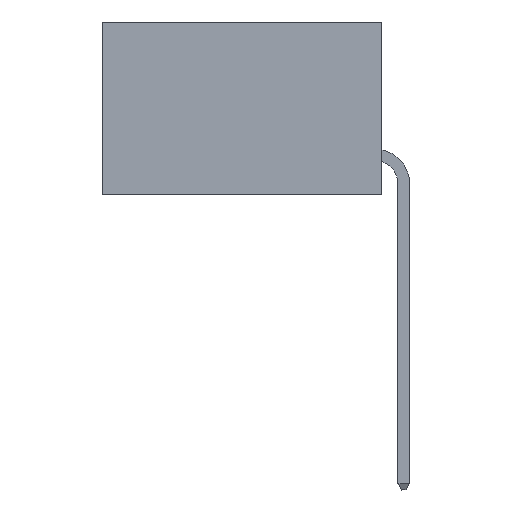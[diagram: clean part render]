
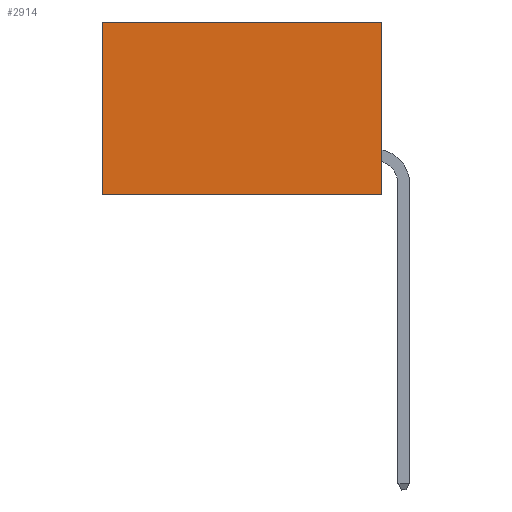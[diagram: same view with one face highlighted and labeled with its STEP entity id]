
A CAD part, left-side view. The second image highlights one B-rep face of the part: STEP entity #2914.
In plain terms, the highlighted planar face has unit normal (-1, 0, 0).
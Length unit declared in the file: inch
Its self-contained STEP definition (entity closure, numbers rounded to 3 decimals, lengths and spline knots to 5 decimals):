
#432 = DIRECTION ( 'NONE',  ( 0., 0., -1. ) ) ;
#879 = VECTOR ( 'NONE', #12371, 39.37008 ) ;
#1306 = VERTEX_POINT ( 'NONE', #19368 ) ;
#1781 = CARTESIAN_POINT ( 'NONE',  ( 0.2875, 0., 0. ) ) ;
#2914 = ADVANCED_FACE ( 'NONE', ( #8203 ), #13613, .F. ) ;
#4081 = AXIS2_PLACEMENT_3D ( 'NONE', #15266, #18232, #9969 ) ;
#5824 = LINE ( 'NONE', #1781, #879 ) ;
#6468 = LINE ( 'NONE', #19767, #13202 ) ;
#6925 = LINE ( 'NONE', #17919, #7445 ) ;
#6989 = VECTOR ( 'NONE', #13274, 39.37008 ) ;
#7445 = VECTOR ( 'NONE', #432, 39.37008 ) ;
#7470 = EDGE_CURVE ( 'NONE', #7918, #1306, #6468, .T. ) ;
#7501 = ORIENTED_EDGE ( 'NONE', *, *, #7470, .T. ) ;
#7918 = VERTEX_POINT ( 'NONE', #10115 ) ;
#8068 = CARTESIAN_POINT ( 'NONE',  ( 0.2875, 0.6, -0.37 ) ) ;
#8203 = FACE_OUTER_BOUND ( 'NONE', #14188, .T. ) ;
#9969 = DIRECTION ( 'NONE',  ( 0., 0., -1. ) ) ;
#10115 = CARTESIAN_POINT ( 'NONE',  ( 0.2875, 0., 0. ) ) ;
#10851 = EDGE_CURVE ( 'NONE', #1306, #10985, #6925, .T. ) ;
#10985 = VERTEX_POINT ( 'NONE', #8068 ) ;
#11368 = LINE ( 'NONE', #20049, #6989 ) ;
#11842 = EDGE_CURVE ( 'NONE', #7918, #19031, #5824, .T. ) ;
#12371 = DIRECTION ( 'NONE',  ( 0., 0., -1. ) ) ;
#13202 = VECTOR ( 'NONE', #18328, 39.37008 ) ;
#13274 = DIRECTION ( 'NONE',  ( 0., 1., 0. ) ) ;
#13613 = PLANE ( 'NONE',  #4081 ) ;
#14188 = EDGE_LOOP ( 'NONE', ( #14488, #14439, #19816, #7501 ) ) ;
#14408 = CARTESIAN_POINT ( 'NONE',  ( 0.2875, 0., -0.37 ) ) ;
#14439 = ORIENTED_EDGE ( 'NONE', *, *, #20379, .F. ) ;
#14488 = ORIENTED_EDGE ( 'NONE', *, *, #10851, .T. ) ;
#15266 = CARTESIAN_POINT ( 'NONE',  ( 0.2875, 0., 0. ) ) ;
#17919 = CARTESIAN_POINT ( 'NONE',  ( 0.2875, 0.6, 0. ) ) ;
#18232 = DIRECTION ( 'NONE',  ( 1., 0., 0. ) ) ;
#18328 = DIRECTION ( 'NONE',  ( 0., 1., 0. ) ) ;
#19031 = VERTEX_POINT ( 'NONE', #14408 ) ;
#19368 = CARTESIAN_POINT ( 'NONE',  ( 0.2875, 0.6, 0. ) ) ;
#19767 = CARTESIAN_POINT ( 'NONE',  ( 0.2875, 0., 0. ) ) ;
#19816 = ORIENTED_EDGE ( 'NONE', *, *, #11842, .F. ) ;
#20049 = CARTESIAN_POINT ( 'NONE',  ( 0.2875, 0., -0.37 ) ) ;
#20379 = EDGE_CURVE ( 'NONE', #19031, #10985, #11368, .T. ) ;
